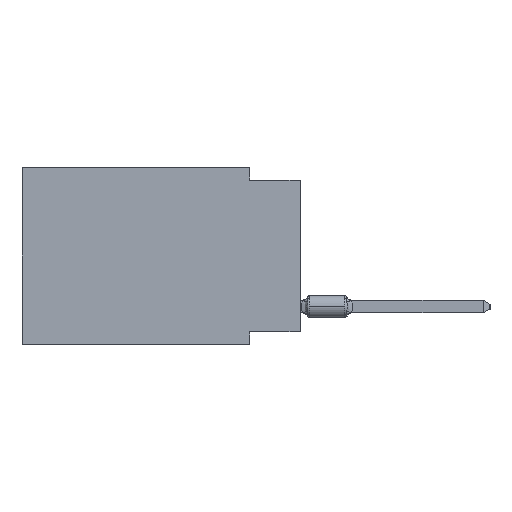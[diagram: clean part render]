
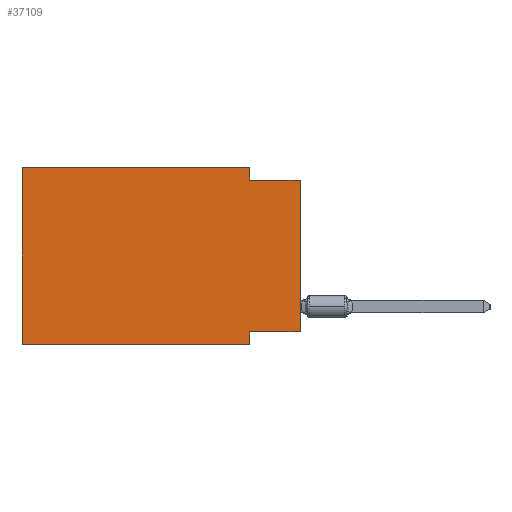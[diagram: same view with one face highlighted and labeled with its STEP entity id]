
A CAD part, left-side view. The second image highlights one B-rep face of the part: STEP entity #37109.
In plain terms, the highlighted planar face has unit normal (-1, 0, 0).
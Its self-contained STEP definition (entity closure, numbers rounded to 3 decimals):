
#395 = CARTESIAN_POINT ( 'NONE',  ( 0., 0., -0.635 ) ) ;
#515 = CARTESIAN_POINT ( 'NONE',  ( 0., 2.54, -8.255 ) ) ;
#1349 = ORIENTED_EDGE ( 'NONE', *, *, #66354, .F. ) ;
#3027 = VECTOR ( 'NONE', #35850, 1000. ) ;
#4414 = VECTOR ( 'NONE', #87638, 1000. ) ;
#4812 = DIRECTION ( 'NONE',  ( 1., 0., 0. ) ) ;
#4822 = CARTESIAN_POINT ( 'NONE',  ( 0., 13.97, -8.89 ) ) ;
#5194 = VECTOR ( 'NONE', #84662, 1000. ) ;
#10776 = EDGE_CURVE ( 'NONE', #40367, #21154, #77533, .T. ) ;
#11264 = LINE ( 'NONE', #27814, #3027 ) ;
#13167 = DIRECTION ( 'NONE',  ( 0., 1., 0. ) ) ;
#16726 = AXIS2_PLACEMENT_3D ( 'NONE', #39006, #4812, #95119 ) ;
#17163 = ORIENTED_EDGE ( 'NONE', *, *, #85158, .F. ) ;
#17477 = VERTEX_POINT ( 'NONE', #62926 ) ;
#21154 = VERTEX_POINT ( 'NONE', #82407 ) ;
#24217 = VERTEX_POINT ( 'NONE', #86498 ) ;
#24969 = DIRECTION ( 'NONE',  ( 0., -1., 0. ) ) ;
#26081 = ORIENTED_EDGE ( 'NONE', *, *, #36959, .T. ) ;
#26437 = LINE ( 'NONE', #60620, #96379 ) ;
#26722 = CARTESIAN_POINT ( 'NONE',  ( 0., 0., -0.635 ) ) ;
#27463 = CARTESIAN_POINT ( 'NONE',  ( 0., 0., -8.255 ) ) ;
#27814 = CARTESIAN_POINT ( 'NONE',  ( 0., 0., 0. ) ) ;
#28904 = LINE ( 'NONE', #70057, #65169 ) ;
#29054 = DIRECTION ( 'NONE',  ( 0., 0., -1. ) ) ;
#32567 = EDGE_CURVE ( 'NONE', #24217, #17477, #28904, .T. ) ;
#34054 = ORIENTED_EDGE ( 'NONE', *, *, #96701, .F. ) ;
#35850 = DIRECTION ( 'NONE',  ( 0., 0., 1. ) ) ;
#36959 = EDGE_CURVE ( 'NONE', #85217, #67475, #11264, .T. ) ;
#37109 = ADVANCED_FACE ( 'NONE', ( #63581 ), #103133, .F. ) ;
#38193 = VERTEX_POINT ( 'NONE', #90927 ) ;
#39006 = CARTESIAN_POINT ( 'NONE',  ( 0., 13.97, 0. ) ) ;
#40367 = VERTEX_POINT ( 'NONE', #96974 ) ;
#42872 = VECTOR ( 'NONE', #24969, 1000. ) ;
#49031 = VECTOR ( 'NONE', #96131, 1000. ) ;
#49597 = CARTESIAN_POINT ( 'NONE',  ( 0., 13.97, 0. ) ) ;
#55650 = ORIENTED_EDGE ( 'NONE', *, *, #32567, .F. ) ;
#55832 = EDGE_CURVE ( 'NONE', #40367, #38193, #105693, .T. ) ;
#60620 = CARTESIAN_POINT ( 'NONE',  ( 0., 2.54, -8.89 ) ) ;
#61633 = VECTOR ( 'NONE', #13167, 1000. ) ;
#62926 = CARTESIAN_POINT ( 'NONE',  ( 0., 2.54, -0.635 ) ) ;
#63581 = FACE_OUTER_BOUND ( 'NONE', #102969, .T. ) ;
#63800 = ORIENTED_EDGE ( 'NONE', *, *, #68636, .F. ) ;
#65169 = VECTOR ( 'NONE', #102643, 1000. ) ;
#66354 = EDGE_CURVE ( 'NONE', #85217, #101947, #76292, .T. ) ;
#67475 = VERTEX_POINT ( 'NONE', #26722 ) ;
#68636 = EDGE_CURVE ( 'NONE', #101947, #21154, #26437, .T. ) ;
#70057 = CARTESIAN_POINT ( 'NONE',  ( 0., 2.54, 0. ) ) ;
#73611 = LINE ( 'NONE', #395, #42872 ) ;
#76292 = LINE ( 'NONE', #94408, #61633 ) ;
#76424 = ORIENTED_EDGE ( 'NONE', *, *, #55832, .F. ) ;
#76644 = LINE ( 'NONE', #85703, #5194 ) ;
#77533 = LINE ( 'NONE', #4822, #4414 ) ;
#79398 = ORIENTED_EDGE ( 'NONE', *, *, #10776, .T. ) ;
#82407 = CARTESIAN_POINT ( 'NONE',  ( 0., 2.54, -8.89 ) ) ;
#84662 = DIRECTION ( 'NONE',  ( 0., -1., 0. ) ) ;
#85158 = EDGE_CURVE ( 'NONE', #38193, #24217, #76644, .T. ) ;
#85217 = VERTEX_POINT ( 'NONE', #27463 ) ;
#85703 = CARTESIAN_POINT ( 'NONE',  ( 0., 13.97, 0. ) ) ;
#86498 = CARTESIAN_POINT ( 'NONE',  ( 0., 2.54, 0. ) ) ;
#87638 = DIRECTION ( 'NONE',  ( 0., -1., 0. ) ) ;
#90927 = CARTESIAN_POINT ( 'NONE',  ( 0., 13.97, 0. ) ) ;
#94408 = CARTESIAN_POINT ( 'NONE',  ( 0., 0., -8.255 ) ) ;
#95119 = DIRECTION ( 'NONE',  ( 0., 0., -1. ) ) ;
#96131 = DIRECTION ( 'NONE',  ( 0., 0., 1. ) ) ;
#96379 = VECTOR ( 'NONE', #29054, 1000. ) ;
#96701 = EDGE_CURVE ( 'NONE', #17477, #67475, #73611, .T. ) ;
#96974 = CARTESIAN_POINT ( 'NONE',  ( 0., 13.97, -8.89 ) ) ;
#101947 = VERTEX_POINT ( 'NONE', #515 ) ;
#102643 = DIRECTION ( 'NONE',  ( 0., 0., -1. ) ) ;
#102969 = EDGE_LOOP ( 'NONE', ( #26081, #34054, #55650, #17163, #76424, #79398, #63800, #1349 ) ) ;
#103133 = PLANE ( 'NONE',  #16726 ) ;
#105693 = LINE ( 'NONE', #49597, #49031 ) ;
